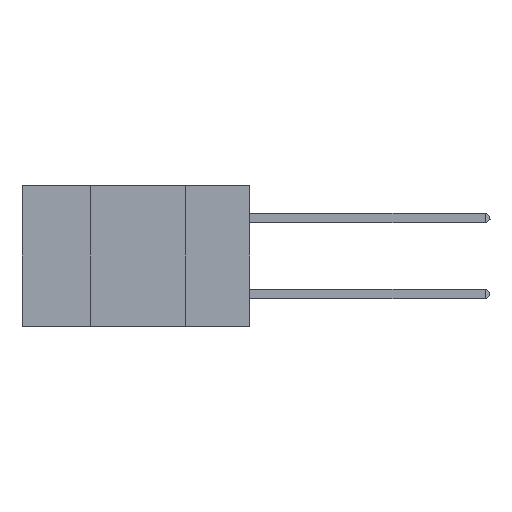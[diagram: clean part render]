
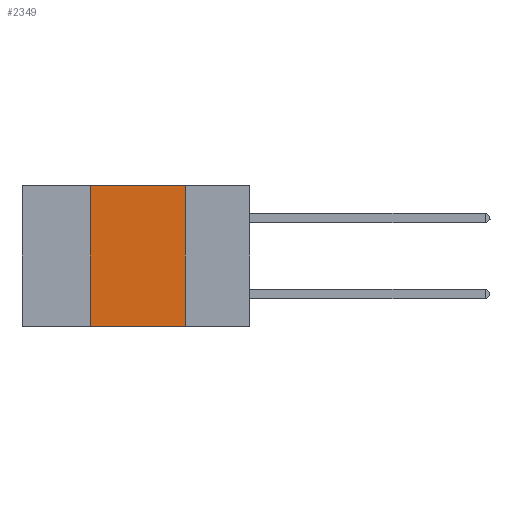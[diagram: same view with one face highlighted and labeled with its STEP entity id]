
A CAD part, left-side view. The second image highlights one B-rep face of the part: STEP entity #2349.
In plain terms, the highlighted planar face has unit normal (-1, 0, 0).
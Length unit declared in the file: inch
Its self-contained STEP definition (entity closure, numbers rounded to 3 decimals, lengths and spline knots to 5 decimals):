
#344 = LINE ( 'NONE', #9219, #7906 ) ;
#2114 = DIRECTION ( 'NONE',  ( 1., 0., 0. ) ) ;
#2349 = ADVANCED_FACE ( 'NONE', ( #10872 ), #15996, .F. ) ;
#2744 = EDGE_CURVE ( 'NONE', #16519, #12679, #344, .T. ) ;
#3607 = DIRECTION ( 'NONE',  ( 0., -1., 0. ) ) ;
#3702 = DIRECTION ( 'NONE',  ( 0., 0., -1. ) ) ;
#4713 = CARTESIAN_POINT ( 'NONE',  ( 0., 0.17, 0. ) ) ;
#5299 = CARTESIAN_POINT ( 'NONE',  ( 0., 0.42, -0.37 ) ) ;
#5416 = EDGE_CURVE ( 'NONE', #16519, #18685, #11690, .T. ) ;
#5480 = CARTESIAN_POINT ( 'NONE',  ( 0., 0.42, 0. ) ) ;
#5887 = VERTEX_POINT ( 'NONE', #4713 ) ;
#7123 = LINE ( 'NONE', #19225, #17017 ) ;
#7328 = CARTESIAN_POINT ( 'NONE',  ( 0., 0.17, 0. ) ) ;
#7906 = VECTOR ( 'NONE', #12520, 39.37008 ) ;
#9219 = CARTESIAN_POINT ( 'NONE',  ( 0., 0.6, -0.37 ) ) ;
#10872 = FACE_OUTER_BOUND ( 'NONE', #20264, .T. ) ;
#11690 = LINE ( 'NONE', #18646, #14475 ) ;
#11842 = ORIENTED_EDGE ( 'NONE', *, *, #5416, .F. ) ;
#11918 = VECTOR ( 'NONE', #14270, 39.37008 ) ;
#12384 = ORIENTED_EDGE ( 'NONE', *, *, #14064, .F. ) ;
#12520 = DIRECTION ( 'NONE',  ( 0., -1., 0. ) ) ;
#12679 = VERTEX_POINT ( 'NONE', #19411 ) ;
#14064 = EDGE_CURVE ( 'NONE', #5887, #12679, #17479, .T. ) ;
#14270 = DIRECTION ( 'NONE',  ( 0., 0., -1. ) ) ;
#14475 = VECTOR ( 'NONE', #22270, 39.37008 ) ;
#15996 = PLANE ( 'NONE',  #16621 ) ;
#16519 = VERTEX_POINT ( 'NONE', #5299 ) ;
#16621 = AXIS2_PLACEMENT_3D ( 'NONE', #17706, #2114, #3702 ) ;
#17017 = VECTOR ( 'NONE', #3607, 39.37008 ) ;
#17479 = LINE ( 'NONE', #7328, #11918 ) ;
#17706 = CARTESIAN_POINT ( 'NONE',  ( 0., 0.6, 0. ) ) ;
#18646 = CARTESIAN_POINT ( 'NONE',  ( 0., 0.42, 0. ) ) ;
#18685 = VERTEX_POINT ( 'NONE', #5480 ) ;
#19225 = CARTESIAN_POINT ( 'NONE',  ( 0., 0.6, 0. ) ) ;
#19411 = CARTESIAN_POINT ( 'NONE',  ( 0., 0.17, -0.37 ) ) ;
#19733 = ORIENTED_EDGE ( 'NONE', *, *, #2744, .T. ) ;
#20264 = EDGE_LOOP ( 'NONE', ( #12384, #20499, #11842, #19733 ) ) ;
#20499 = ORIENTED_EDGE ( 'NONE', *, *, #21249, .F. ) ;
#21249 = EDGE_CURVE ( 'NONE', #18685, #5887, #7123, .T. ) ;
#22270 = DIRECTION ( 'NONE',  ( 0., 0., 1. ) ) ;
